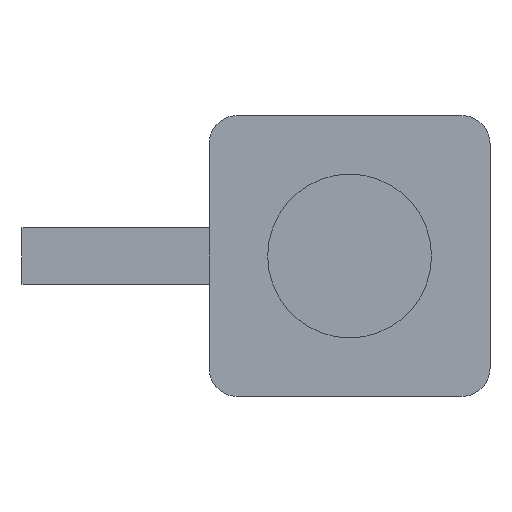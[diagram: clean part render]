
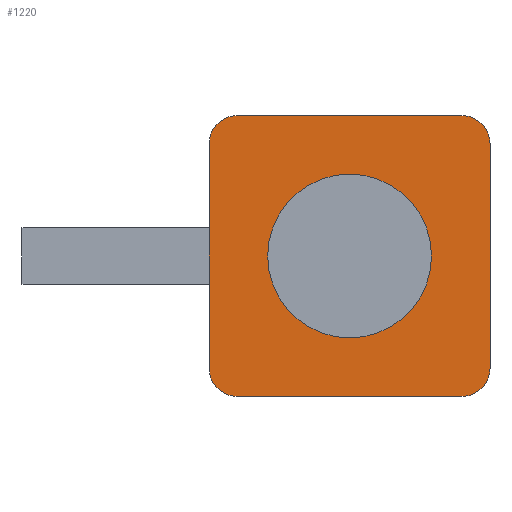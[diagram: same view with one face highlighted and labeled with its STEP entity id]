
A CAD part, front view. The second image highlights one B-rep face of the part: STEP entity #1220.
In plain terms, the highlighted planar face has unit normal (0, -1, 0).
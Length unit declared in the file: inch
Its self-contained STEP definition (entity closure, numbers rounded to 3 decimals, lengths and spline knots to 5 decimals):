
#7 = LINE ( 'NONE', #648, #1512 ) ;
#26 = LINE ( 'NONE', #789, #1353 ) ;
#29 = EDGE_LOOP ( 'NONE', ( #2005, #1159 ) ) ;
#38 = VERTEX_POINT ( 'NONE', #50 ) ;
#47 = AXIS2_PLACEMENT_3D ( 'NONE', #186, #1465, #2098 ) ;
#50 = CARTESIAN_POINT ( 'NONE',  ( 0., -2.8, 1.35 ) ) ;
#65 = CARTESIAN_POINT ( 'NONE',  ( 1.5, -2.8, 0. ) ) ;
#106 = DIRECTION ( 'NONE',  ( 0., -1., 0. ) ) ;
#125 = ORIENTED_EDGE ( 'NONE', *, *, #1475, .T. ) ;
#142 = CARTESIAN_POINT ( 'NONE',  ( 1.35, -2.8, 0.15 ) ) ;
#152 = DIRECTION ( 'NONE',  ( 0., -1., 0. ) ) ;
#164 = FACE_BOUND ( 'NONE', #29, .T. ) ;
#186 = CARTESIAN_POINT ( 'NONE',  ( 0.75, -2.8, 0.75 ) ) ;
#221 = EDGE_CURVE ( 'NONE', #1114, #1848, #1177, .T. ) ;
#232 = ORIENTED_EDGE ( 'NONE', *, *, #336, .T. ) ;
#238 = VERTEX_POINT ( 'NONE', #1097 ) ;
#264 = EDGE_CURVE ( 'NONE', #1040, #238, #1669, .T. ) ;
#286 = ORIENTED_EDGE ( 'NONE', *, *, #221, .T. ) ;
#302 = DIRECTION ( 'NONE',  ( 0., -1., 0. ) ) ;
#316 = FACE_OUTER_BOUND ( 'NONE', #1043, .T. ) ;
#336 = EDGE_CURVE ( 'NONE', #1453, #1114, #7, .T. ) ;
#385 = AXIS2_PLACEMENT_3D ( 'NONE', #1687, #1345, #2004 ) ;
#469 = CIRCLE ( 'NONE', #385, 0.15 ) ;
#490 = VERTEX_POINT ( 'NONE', #547 ) ;
#547 = CARTESIAN_POINT ( 'NONE',  ( 1.35, -2.8, 1.5 ) ) ;
#568 = DIRECTION ( 'NONE',  ( 0., 0., 1. ) ) ;
#590 = CARTESIAN_POINT ( 'NONE',  ( 1.5, -2.8, 0.15 ) ) ;
#642 = AXIS2_PLACEMENT_3D ( 'NONE', #1670, #2023, #1050 ) ;
#648 = CARTESIAN_POINT ( 'NONE',  ( 0., -2.8, 0. ) ) ;
#694 = LINE ( 'NONE', #1060, #1866 ) ;
#766 = CARTESIAN_POINT ( 'NONE',  ( 0.75, -2.8, 0.3125 ) ) ;
#789 = CARTESIAN_POINT ( 'NONE',  ( 0., -2.8, 1.5 ) ) ;
#804 = EDGE_CURVE ( 'NONE', #1848, #1184, #1586, .T. ) ;
#839 = ORIENTED_EDGE ( 'NONE', *, *, #903, .T. ) ;
#844 = DIRECTION ( 'NONE',  ( 1., 0., 0. ) ) ;
#892 = DIRECTION ( 'NONE',  ( 0., 0., -1. ) ) ;
#903 = EDGE_CURVE ( 'NONE', #1090, #38, #955, .T. ) ;
#949 = ORIENTED_EDGE ( 'NONE', *, *, #1910, .T. ) ;
#955 = CIRCLE ( 'NONE', #642, 0.15 ) ;
#992 = PLANE ( 'NONE',  #1644 ) ;
#1011 = EDGE_CURVE ( 'NONE', #38, #1784, #694, .T. ) ;
#1040 = VERTEX_POINT ( 'NONE', #766 ) ;
#1043 = EDGE_LOOP ( 'NONE', ( #286, #1425, #949, #1471, #839, #1134, #125, #232 ) ) ;
#1050 = DIRECTION ( 'NONE',  ( 0., 0., -1. ) ) ;
#1060 = CARTESIAN_POINT ( 'NONE',  ( 0., -2.8, 0. ) ) ;
#1090 = VERTEX_POINT ( 'NONE', #1751 ) ;
#1097 = CARTESIAN_POINT ( 'NONE',  ( 0.75, -2.8, 1.1875 ) ) ;
#1104 = CARTESIAN_POINT ( 'NONE',  ( 1.35, -2.8, 0. ) ) ;
#1108 = EDGE_CURVE ( 'NONE', #490, #1090, #26, .T. ) ;
#1114 = VERTEX_POINT ( 'NONE', #1104 ) ;
#1134 = ORIENTED_EDGE ( 'NONE', *, *, #1011, .T. ) ;
#1142 = VECTOR ( 'NONE', #568, 39.37008 ) ;
#1159 = ORIENTED_EDGE ( 'NONE', *, *, #264, .F. ) ;
#1177 = CIRCLE ( 'NONE', #1387, 0.15 ) ;
#1184 = VERTEX_POINT ( 'NONE', #1296 ) ;
#1220 = ADVANCED_FACE ( 'NONE', ( #316, #164 ), #992, .T. ) ;
#1252 = DIRECTION ( 'NONE',  ( 0., 0., -1. ) ) ;
#1275 = DIRECTION ( 'NONE',  ( 0., 0., -1. ) ) ;
#1296 = CARTESIAN_POINT ( 'NONE',  ( 1.5, -2.8, 1.35 ) ) ;
#1345 = DIRECTION ( 'NONE',  ( 0., -1., 0. ) ) ;
#1353 = VECTOR ( 'NONE', #1606, 39.37008 ) ;
#1380 = AXIS2_PLACEMENT_3D ( 'NONE', #1521, #106, #892 ) ;
#1387 = AXIS2_PLACEMENT_3D ( 'NONE', #142, #302, #1252 ) ;
#1425 = ORIENTED_EDGE ( 'NONE', *, *, #804, .T. ) ;
#1453 = VERTEX_POINT ( 'NONE', #2027 ) ;
#1465 = DIRECTION ( 'NONE',  ( 0., -1., 0. ) ) ;
#1471 = ORIENTED_EDGE ( 'NONE', *, *, #1108, .T. ) ;
#1475 = EDGE_CURVE ( 'NONE', #1784, #1453, #469, .T. ) ;
#1512 = VECTOR ( 'NONE', #844, 39.37008 ) ;
#1521 = CARTESIAN_POINT ( 'NONE',  ( 1.35, -2.8, 1.35 ) ) ;
#1586 = LINE ( 'NONE', #65, #1142 ) ;
#1606 = DIRECTION ( 'NONE',  ( -1., 0., 0. ) ) ;
#1610 = DIRECTION ( 'NONE',  ( 0., 0., -1. ) ) ;
#1619 = CARTESIAN_POINT ( 'NONE',  ( 0., -2.8, 0.15 ) ) ;
#1620 = DIRECTION ( 'NONE',  ( 0., -1., 0. ) ) ;
#1644 = AXIS2_PLACEMENT_3D ( 'NONE', #1947, #1620, #1610 ) ;
#1669 = CIRCLE ( 'NONE', #47, 0.4375 ) ;
#1670 = CARTESIAN_POINT ( 'NONE',  ( 0.15, -2.8, 1.35 ) ) ;
#1687 = CARTESIAN_POINT ( 'NONE',  ( 0.15, -2.8, 0.15 ) ) ;
#1740 = AXIS2_PLACEMENT_3D ( 'NONE', #1756, #152, #1275 ) ;
#1751 = CARTESIAN_POINT ( 'NONE',  ( 0.15, -2.8, 1.5 ) ) ;
#1756 = CARTESIAN_POINT ( 'NONE',  ( 0.75, -2.8, 0.75 ) ) ;
#1784 = VERTEX_POINT ( 'NONE', #1619 ) ;
#1848 = VERTEX_POINT ( 'NONE', #590 ) ;
#1866 = VECTOR ( 'NONE', #2048, 39.37008 ) ;
#1896 = CIRCLE ( 'NONE', #1380, 0.15 ) ;
#1910 = EDGE_CURVE ( 'NONE', #1184, #490, #1896, .T. ) ;
#1947 = CARTESIAN_POINT ( 'NONE',  ( 0., -2.8, 0. ) ) ;
#1992 = CIRCLE ( 'NONE', #1740, 0.4375 ) ;
#2004 = DIRECTION ( 'NONE',  ( 0., 0., -1. ) ) ;
#2005 = ORIENTED_EDGE ( 'NONE', *, *, #2050, .F. ) ;
#2023 = DIRECTION ( 'NONE',  ( 0., -1., 0. ) ) ;
#2027 = CARTESIAN_POINT ( 'NONE',  ( 0.15, -2.8, 0. ) ) ;
#2048 = DIRECTION ( 'NONE',  ( 0., 0., -1. ) ) ;
#2050 = EDGE_CURVE ( 'NONE', #238, #1040, #1992, .T. ) ;
#2098 = DIRECTION ( 'NONE',  ( 0., 0., -1. ) ) ;
